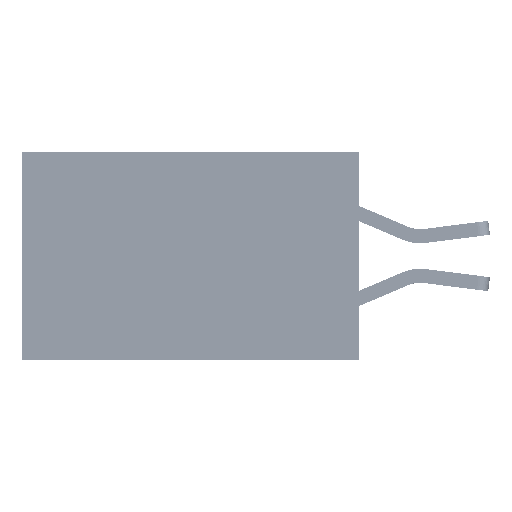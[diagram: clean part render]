
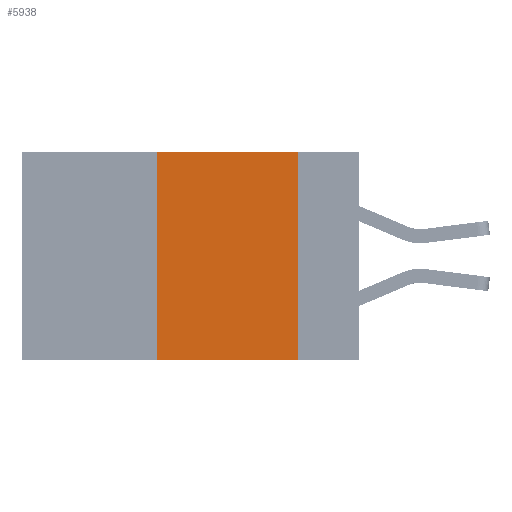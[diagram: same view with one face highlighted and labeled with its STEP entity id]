
A CAD part, left-side view. The second image highlights one B-rep face of the part: STEP entity #5938.
In plain terms, the highlighted planar face has unit normal (-1, 0, 0).
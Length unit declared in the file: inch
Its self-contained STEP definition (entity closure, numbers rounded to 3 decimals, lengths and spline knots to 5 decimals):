
#3531 = FACE_OUTER_BOUND ( 'NONE', #13756, .T. ) ;
#3608 = DIRECTION ( 'NONE',  ( 0., 0., 1. ) ) ;
#3630 = LINE ( 'NONE', #27942, #12317 ) ;
#3980 = AXIS2_PLACEMENT_3D ( 'NONE', #39645, #19937, #16326 ) ;
#4105 = VECTOR ( 'NONE', #14316, 39.37008 ) ;
#5938 = ADVANCED_FACE ( 'NONE', ( #3531 ), #20077, .F. ) ;
#7278 = CARTESIAN_POINT ( 'NONE',  ( 0., 0.36, 0. ) ) ;
#9558 = EDGE_CURVE ( 'NONE', #36122, #41225, #22706, .T. ) ;
#12264 = LINE ( 'NONE', #40472, #4105 ) ;
#12317 = VECTOR ( 'NONE', #27516, 39.37008 ) ;
#12579 = EDGE_CURVE ( 'NONE', #14038, #28706, #12264, .T. ) ;
#13715 = VECTOR ( 'NONE', #3608, 39.37008 ) ;
#13756 = EDGE_LOOP ( 'NONE', ( #37563, #38635, #37346, #38829 ) ) ;
#14038 = VERTEX_POINT ( 'NONE', #22592 ) ;
#14316 = DIRECTION ( 'NONE',  ( 0., -1., 0. ) ) ;
#15756 = LINE ( 'NONE', #36059, #13715 ) ;
#16326 = DIRECTION ( 'NONE',  ( 0., 0., -1. ) ) ;
#19937 = DIRECTION ( 'NONE',  ( 1., 0., 0. ) ) ;
#20077 = PLANE ( 'NONE',  #3980 ) ;
#20761 = CARTESIAN_POINT ( 'NONE',  ( 0., 0.11, -0.37 ) ) ;
#22592 = CARTESIAN_POINT ( 'NONE',  ( 0., 0.36, -0.37 ) ) ;
#22706 = LINE ( 'NONE', #24629, #41196 ) ;
#24034 = CARTESIAN_POINT ( 'NONE',  ( 0., 0.11, 0. ) ) ;
#24629 = CARTESIAN_POINT ( 'NONE',  ( 0., 0.6, 0. ) ) ;
#27516 = DIRECTION ( 'NONE',  ( 0., 0., -1. ) ) ;
#27942 = CARTESIAN_POINT ( 'NONE',  ( 0., 0.11, 0. ) ) ;
#28079 = EDGE_CURVE ( 'NONE', #41225, #28706, #3630, .T. ) ;
#28706 = VERTEX_POINT ( 'NONE', #20761 ) ;
#36059 = CARTESIAN_POINT ( 'NONE',  ( 0., 0.36, 0. ) ) ;
#36122 = VERTEX_POINT ( 'NONE', #7278 ) ;
#37346 = ORIENTED_EDGE ( 'NONE', *, *, #38037, .F. ) ;
#37563 = ORIENTED_EDGE ( 'NONE', *, *, #28079, .F. ) ;
#37897 = DIRECTION ( 'NONE',  ( 0., -1., 0. ) ) ;
#38037 = EDGE_CURVE ( 'NONE', #14038, #36122, #15756, .T. ) ;
#38635 = ORIENTED_EDGE ( 'NONE', *, *, #9558, .F. ) ;
#38829 = ORIENTED_EDGE ( 'NONE', *, *, #12579, .T. ) ;
#39645 = CARTESIAN_POINT ( 'NONE',  ( 0., 0.6, 0. ) ) ;
#40472 = CARTESIAN_POINT ( 'NONE',  ( 0., 0.6, -0.37 ) ) ;
#41196 = VECTOR ( 'NONE', #37897, 39.37008 ) ;
#41225 = VERTEX_POINT ( 'NONE', #24034 ) ;
